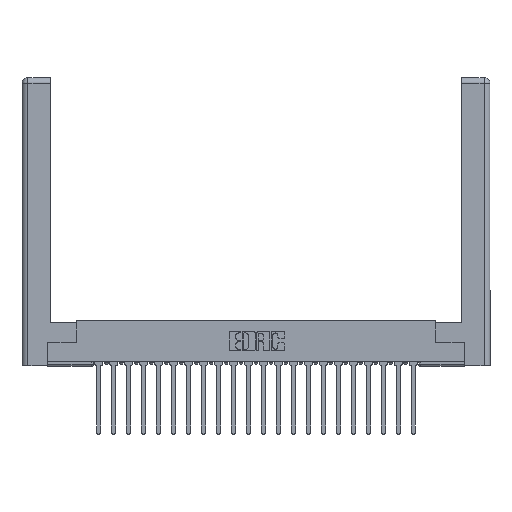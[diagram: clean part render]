
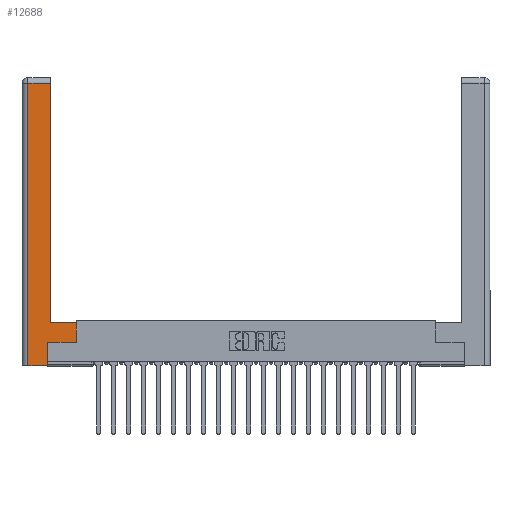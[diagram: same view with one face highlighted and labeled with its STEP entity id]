
A CAD part, top view. The second image highlights one B-rep face of the part: STEP entity #12688.
In plain terms, the highlighted planar face has unit normal (0, 0, 1).
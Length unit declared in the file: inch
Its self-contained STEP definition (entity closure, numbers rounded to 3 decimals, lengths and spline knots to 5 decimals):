
#149 = CARTESIAN_POINT ( 'NONE',  ( 0.265, 0., 0. ) ) ;
#372 = LINE ( 'NONE', #20473, #23549 ) ;
#862 = LINE ( 'NONE', #16398, #21986 ) ;
#1391 = VERTEX_POINT ( 'NONE', #4893 ) ;
#1526 = EDGE_CURVE ( 'NONE', #18260, #17513, #862, .T. ) ;
#1984 = DIRECTION ( 'NONE',  ( 1., 0., 0. ) ) ;
#2188 = CARTESIAN_POINT ( 'NONE',  ( 0., 0., 0. ) ) ;
#3013 = CARTESIAN_POINT ( 'NONE',  ( 0.295, 0.45, 0. ) ) ;
#3504 = DIRECTION ( 'NONE',  ( 0., 1., 0. ) ) ;
#3905 = LINE ( 'NONE', #9421, #14921 ) ;
#4306 = PLANE ( 'NONE',  #17741 ) ;
#4862 = EDGE_LOOP ( 'NONE', ( #22913, #8566, #22925, #23260, #8888, #14842, #7098, #6949 ) ) ;
#4893 = CARTESIAN_POINT ( 'NONE',  ( 0.295, 2.94, 0. ) ) ;
#5746 = DIRECTION ( 'NONE',  ( -1., 0., 0. ) ) ;
#5753 = EDGE_CURVE ( 'NONE', #1391, #12536, #9765, .T. ) ;
#6075 = VERTEX_POINT ( 'NONE', #12199 ) ;
#6157 = CARTESIAN_POINT ( 'NONE',  ( 0.565, 0.45, 0. ) ) ;
#6949 = ORIENTED_EDGE ( 'NONE', *, *, #13883, .T. ) ;
#7098 = ORIENTED_EDGE ( 'NONE', *, *, #15276, .T. ) ;
#7146 = VERTEX_POINT ( 'NONE', #22471 ) ;
#7308 = LINE ( 'NONE', #6157, #10524 ) ;
#7607 = DIRECTION ( 'NONE',  ( 0., 1., 0. ) ) ;
#7814 = LINE ( 'NONE', #20118, #8415 ) ;
#8026 = DIRECTION ( 'NONE',  ( 0., 1., 0. ) ) ;
#8415 = VECTOR ( 'NONE', #3504, 39.37008 ) ;
#8566 = ORIENTED_EDGE ( 'NONE', *, *, #5753, .T. ) ;
#8876 = CARTESIAN_POINT ( 'NONE',  ( 0.0615, 2.94, 0. ) ) ;
#8888 = ORIENTED_EDGE ( 'NONE', *, *, #22420, .T. ) ;
#9421 = CARTESIAN_POINT ( 'NONE',  ( 0.295, 0.45, 0. ) ) ;
#9765 = LINE ( 'NONE', #22657, #21645 ) ;
#10524 = VECTOR ( 'NONE', #8026, 39.37008 ) ;
#10558 = LINE ( 'NONE', #16777, #13413 ) ;
#10993 = EDGE_CURVE ( 'NONE', #22684, #1391, #7814, .T. ) ;
#11101 = LINE ( 'NONE', #149, #20397 ) ;
#12199 = CARTESIAN_POINT ( 'NONE',  ( 0.0615, 0., 0. ) ) ;
#12536 = VERTEX_POINT ( 'NONE', #8876 ) ;
#12688 = ADVANCED_FACE ( 'NONE', ( #21951 ), #4306, .F. ) ;
#13413 = VECTOR ( 'NONE', #7607, 39.37008 ) ;
#13423 = DIRECTION ( 'NONE',  ( 0., 0., -1. ) ) ;
#13486 = CARTESIAN_POINT ( 'NONE',  ( 0.265, 0.245, 0. ) ) ;
#13883 = EDGE_CURVE ( 'NONE', #7146, #22684, #3905, .T. ) ;
#14842 = ORIENTED_EDGE ( 'NONE', *, *, #1526, .T. ) ;
#14921 = VECTOR ( 'NONE', #20056, 39.37008 ) ;
#15002 = EDGE_CURVE ( 'NONE', #12536, #6075, #372, .T. ) ;
#15004 = EDGE_CURVE ( 'NONE', #6075, #18111, #11101, .T. ) ;
#15276 = EDGE_CURVE ( 'NONE', #17513, #7146, #7308, .T. ) ;
#16398 = CARTESIAN_POINT ( 'NONE',  ( 0.565, 0.245, 0. ) ) ;
#16777 = CARTESIAN_POINT ( 'NONE',  ( 0.265, 0.245, 0. ) ) ;
#16921 = CARTESIAN_POINT ( 'NONE',  ( 0.265, 0., 0. ) ) ;
#17346 = DIRECTION ( 'NONE',  ( -1., 0., 0. ) ) ;
#17513 = VERTEX_POINT ( 'NONE', #23653 ) ;
#17741 = AXIS2_PLACEMENT_3D ( 'NONE', #2188, #13423, #5746 ) ;
#18111 = VERTEX_POINT ( 'NONE', #16921 ) ;
#18260 = VERTEX_POINT ( 'NONE', #13486 ) ;
#20056 = DIRECTION ( 'NONE',  ( -1., 0., 0. ) ) ;
#20118 = CARTESIAN_POINT ( 'NONE',  ( 0.295, 3., 0. ) ) ;
#20397 = VECTOR ( 'NONE', #1984, 39.37008 ) ;
#20473 = CARTESIAN_POINT ( 'NONE',  ( 0.0615, 0., 0. ) ) ;
#21645 = VECTOR ( 'NONE', #17346, 39.37008 ) ;
#21951 = FACE_OUTER_BOUND ( 'NONE', #4862, .T. ) ;
#21986 = VECTOR ( 'NONE', #23638, 39.37008 ) ;
#22291 = DIRECTION ( 'NONE',  ( 0., -1., 0. ) ) ;
#22420 = EDGE_CURVE ( 'NONE', #18111, #18260, #10558, .T. ) ;
#22471 = CARTESIAN_POINT ( 'NONE',  ( 0.565, 0.45, 0. ) ) ;
#22657 = CARTESIAN_POINT ( 'NONE',  ( 0.0615, 2.94, 0. ) ) ;
#22684 = VERTEX_POINT ( 'NONE', #3013 ) ;
#22913 = ORIENTED_EDGE ( 'NONE', *, *, #10993, .T. ) ;
#22925 = ORIENTED_EDGE ( 'NONE', *, *, #15002, .T. ) ;
#23260 = ORIENTED_EDGE ( 'NONE', *, *, #15004, .T. ) ;
#23549 = VECTOR ( 'NONE', #22291, 39.37008 ) ;
#23638 = DIRECTION ( 'NONE',  ( 1., 0., 0. ) ) ;
#23653 = CARTESIAN_POINT ( 'NONE',  ( 0.565, 0.245, 0. ) ) ;
